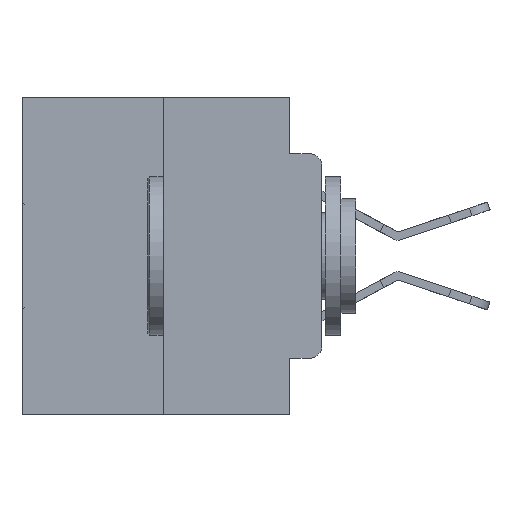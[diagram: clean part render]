
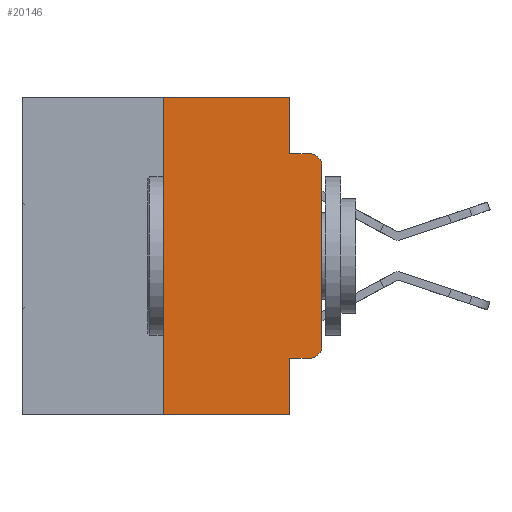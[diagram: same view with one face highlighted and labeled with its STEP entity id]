
A CAD part, left-side view. The second image highlights one B-rep face of the part: STEP entity #20146.
In plain terms, the highlighted planar face has unit normal (-1, 0, 0).
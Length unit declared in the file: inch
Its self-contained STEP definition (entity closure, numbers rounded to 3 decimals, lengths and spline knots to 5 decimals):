
#216 = ORIENTED_EDGE ( 'NONE', *, *, #25261, .T. ) ;
#325 = AXIS2_PLACEMENT_3D ( 'NONE', #24724, #12660, #29580 ) ;
#352 = CARTESIAN_POINT ( 'NONE',  ( 0., 0.051, -0.5 ) ) ;
#557 = DIRECTION ( 'NONE',  ( 0., -1., 0. ) ) ;
#800 = CARTESIAN_POINT ( 'NONE',  ( 0., 0., 0. ) ) ;
#1036 = VECTOR ( 'NONE', #3388, 39.37008 ) ;
#1096 = CARTESIAN_POINT ( 'NONE',  ( 0., 0.02, -0.0885 ) ) ;
#1378 = VERTEX_POINT ( 'NONE', #4441 ) ;
#1589 = AXIS2_PLACEMENT_3D ( 'NONE', #9094, #26056, #11557 ) ;
#1871 = ORIENTED_EDGE ( 'NONE', *, *, #25764, .T. ) ;
#1998 = CARTESIAN_POINT ( 'NONE',  ( 0., 0.473, 0. ) ) ;
#2262 = ORIENTED_EDGE ( 'NONE', *, *, #14323, .T. ) ;
#2322 = VERTEX_POINT ( 'NONE', #26058 ) ;
#3198 = DIRECTION ( 'NONE',  ( 0., 0., -1. ) ) ;
#3292 = DIRECTION ( 'NONE',  ( 0., 0., -1. ) ) ;
#3388 = DIRECTION ( 'NONE',  ( 0., 0., 1. ) ) ;
#3705 = CARTESIAN_POINT ( 'NONE',  ( 0., 0.473, -0.5 ) ) ;
#4374 = VECTOR ( 'NONE', #557, 39.37008 ) ;
#4441 = CARTESIAN_POINT ( 'NONE',  ( 0., 0.02, -0.4115 ) ) ;
#4548 = DIRECTION ( 'NONE',  ( 0., -1., 0. ) ) ;
#4767 = FACE_OUTER_BOUND ( 'NONE', #26906, .T. ) ;
#4910 = CARTESIAN_POINT ( 'NONE',  ( 0., 0.051, -0.0885 ) ) ;
#5449 = EDGE_CURVE ( 'NONE', #5696, #18696, #14459, .T. ) ;
#5487 = LINE ( 'NONE', #3705, #29012 ) ;
#5608 = CARTESIAN_POINT ( 'NONE',  ( 0., 0.051, -0.4115 ) ) ;
#5696 = VERTEX_POINT ( 'NONE', #6755 ) ;
#6216 = DIRECTION ( 'NONE',  ( 0., -1., 0. ) ) ;
#6755 = CARTESIAN_POINT ( 'NONE',  ( 0., 0.051, 0. ) ) ;
#7468 = EDGE_CURVE ( 'NONE', #21067, #25862, #26862, .T. ) ;
#8981 = VERTEX_POINT ( 'NONE', #352 ) ;
#9094 = CARTESIAN_POINT ( 'NONE',  ( 0., 0.02, -0.1085 ) ) ;
#9627 = ORIENTED_EDGE ( 'NONE', *, *, #7468, .T. ) ;
#9655 = VERTEX_POINT ( 'NONE', #22534 ) ;
#10464 = VECTOR ( 'NONE', #29999, 39.37008 ) ;
#11362 = AXIS2_PLACEMENT_3D ( 'NONE', #27618, #13105, #30022 ) ;
#11557 = DIRECTION ( 'NONE',  ( 0., 0., -1. ) ) ;
#11794 = VECTOR ( 'NONE', #4548, 39.37008 ) ;
#11926 = ORIENTED_EDGE ( 'NONE', *, *, #23591, .F. ) ;
#12299 = VECTOR ( 'NONE', #12849, 39.37008 ) ;
#12534 = EDGE_CURVE ( 'NONE', #19665, #2322, #16859, .T. ) ;
#12660 = DIRECTION ( 'NONE',  ( 1., 0., 0. ) ) ;
#12849 = DIRECTION ( 'NONE',  ( 0., -1., 0. ) ) ;
#13105 = DIRECTION ( 'NONE',  ( -1., 0., 0. ) ) ;
#13423 = ORIENTED_EDGE ( 'NONE', *, *, #22062, .F. ) ;
#14323 = EDGE_CURVE ( 'NONE', #24607, #21067, #14908, .T. ) ;
#14459 = LINE ( 'NONE', #22783, #25851 ) ;
#14908 = LINE ( 'NONE', #800, #1036 ) ;
#15384 = CARTESIAN_POINT ( 'NONE',  ( 0., 0.051, 0. ) ) ;
#15503 = CARTESIAN_POINT ( 'NONE',  ( 0., 0.25, 0. ) ) ;
#15973 = CARTESIAN_POINT ( 'NONE',  ( 0., 0., -0.1085 ) ) ;
#16859 = LINE ( 'NONE', #15503, #10464 ) ;
#18275 = ORIENTED_EDGE ( 'NONE', *, *, #12534, .F. ) ;
#18696 = VERTEX_POINT ( 'NONE', #4910 ) ;
#19665 = VERTEX_POINT ( 'NONE', #29824 ) ;
#19775 = PLANE ( 'NONE',  #325 ) ;
#19784 = ORIENTED_EDGE ( 'NONE', *, *, #26367, .T. ) ;
#20146 = ADVANCED_FACE ( 'NONE', ( #4767 ), #19775, .F. ) ;
#20349 = LINE ( 'NONE', #1998, #11794 ) ;
#21067 = VERTEX_POINT ( 'NONE', #15973 ) ;
#22062 = EDGE_CURVE ( 'NONE', #9655, #8981, #28182, .T. ) ;
#22534 = CARTESIAN_POINT ( 'NONE',  ( 0., 0.051, -0.4115 ) ) ;
#22663 = CARTESIAN_POINT ( 'NONE',  ( 0., 0.051, -0.0885 ) ) ;
#22783 = CARTESIAN_POINT ( 'NONE',  ( 0., 0.051, 0. ) ) ;
#23273 = ORIENTED_EDGE ( 'NONE', *, *, #24570, .F. ) ;
#23591 = EDGE_CURVE ( 'NONE', #2322, #5696, #20349, .T. ) ;
#23759 = LINE ( 'NONE', #22663, #4374 ) ;
#24570 = EDGE_CURVE ( 'NONE', #18696, #25862, #23759, .T. ) ;
#24607 = VERTEX_POINT ( 'NONE', #30059 ) ;
#24724 = CARTESIAN_POINT ( 'NONE',  ( 0., 0.473, 0. ) ) ;
#25261 = EDGE_CURVE ( 'NONE', #19665, #8981, #5487, .T. ) ;
#25764 = EDGE_CURVE ( 'NONE', #1378, #24607, #27486, .T. ) ;
#25851 = VECTOR ( 'NONE', #3292, 39.37008 ) ;
#25862 = VERTEX_POINT ( 'NONE', #1096 ) ;
#26056 = DIRECTION ( 'NONE',  ( -1., 0., 0. ) ) ;
#26058 = CARTESIAN_POINT ( 'NONE',  ( 0., 0.25, 0. ) ) ;
#26367 = EDGE_CURVE ( 'NONE', #9655, #1378, #30071, .T. ) ;
#26862 = CIRCLE ( 'NONE', #1589, 0.02 ) ;
#26906 = EDGE_LOOP ( 'NONE', ( #2262, #9627, #23273, #29700, #11926, #18275, #216, #13423, #19784, #1871 ) ) ;
#27486 = CIRCLE ( 'NONE', #11362, 0.02 ) ;
#27618 = CARTESIAN_POINT ( 'NONE',  ( 0., 0.02, -0.3915 ) ) ;
#28182 = LINE ( 'NONE', #15384, #29686 ) ;
#29012 = VECTOR ( 'NONE', #6216, 39.37008 ) ;
#29580 = DIRECTION ( 'NONE',  ( 0., 0., -1. ) ) ;
#29686 = VECTOR ( 'NONE', #3198, 39.37008 ) ;
#29700 = ORIENTED_EDGE ( 'NONE', *, *, #5449, .F. ) ;
#29824 = CARTESIAN_POINT ( 'NONE',  ( 0., 0.25, -0.5 ) ) ;
#29999 = DIRECTION ( 'NONE',  ( 0., 0., 1. ) ) ;
#30022 = DIRECTION ( 'NONE',  ( 0., 0., -1. ) ) ;
#30059 = CARTESIAN_POINT ( 'NONE',  ( 0., 0., -0.3915 ) ) ;
#30071 = LINE ( 'NONE', #5608, #12299 ) ;
